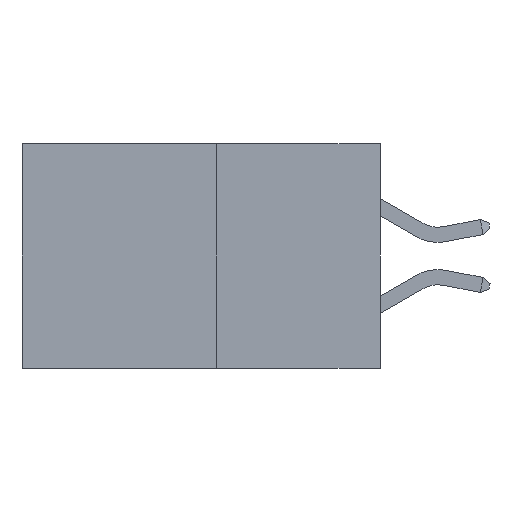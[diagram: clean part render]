
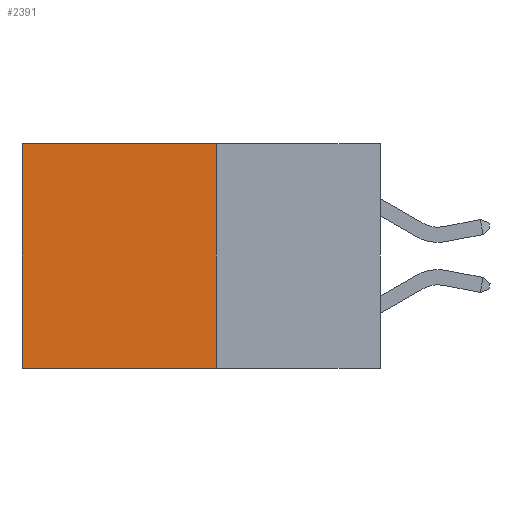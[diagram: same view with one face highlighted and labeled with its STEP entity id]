
A CAD part, left-side view. The second image highlights one B-rep face of the part: STEP entity #2391.
In plain terms, the highlighted planar face has unit normal (-1, 0, 0).
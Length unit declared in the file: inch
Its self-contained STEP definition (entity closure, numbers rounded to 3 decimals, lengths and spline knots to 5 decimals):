
#100 = VERTEX_POINT ( 'NONE', #1561 ) ;
#181 = ORIENTED_EDGE ( 'NONE', *, *, #696, .T. ) ;
#211 = ORIENTED_EDGE ( 'NONE', *, *, #6162, .F. ) ;
#221 = ORIENTED_EDGE ( 'NONE', *, *, #8877, .F. ) ;
#266 = ORIENTED_EDGE ( 'NONE', *, *, #320, .T. ) ;
#320 = EDGE_CURVE ( 'NONE', #9287, #100, #10865, .T. ) ;
#696 = EDGE_CURVE ( 'NONE', #100, #4154, #11442, .T. ) ;
#724 = LINE ( 'NONE', #2511, #7704 ) ;
#786 = VERTEX_POINT ( 'NONE', #1816 ) ;
#1243 = VECTOR ( 'NONE', #10670, 39.37008 ) ;
#1561 = CARTESIAN_POINT ( 'NONE',  ( 0.277, 0.59, 0. ) ) ;
#1816 = CARTESIAN_POINT ( 'NONE',  ( 0.277, 0.27, -0.37 ) ) ;
#2391 = ADVANCED_FACE ( 'NONE', ( #6535 ), #7886, .F. ) ;
#2511 = CARTESIAN_POINT ( 'NONE',  ( 0.277, 0.27, -0.37 ) ) ;
#2722 = DIRECTION ( 'NONE',  ( 1., 0., 0. ) ) ;
#3398 = LINE ( 'NONE', #9887, #5112 ) ;
#3679 = DIRECTION ( 'NONE',  ( 0., 0., -1. ) ) ;
#4154 = VERTEX_POINT ( 'NONE', #10105 ) ;
#5112 = VECTOR ( 'NONE', #10684, 39.37008 ) ;
#5475 = AXIS2_PLACEMENT_3D ( 'NONE', #6475, #2722, #6484 ) ;
#5680 = EDGE_LOOP ( 'NONE', ( #181, #211, #221, #266 ) ) ;
#6162 = EDGE_CURVE ( 'NONE', #786, #4154, #3398, .T. ) ;
#6475 = CARTESIAN_POINT ( 'NONE',  ( 0.277, 0.27, -0.37 ) ) ;
#6484 = DIRECTION ( 'NONE',  ( 0., 0., -1. ) ) ;
#6535 = FACE_OUTER_BOUND ( 'NONE', #5680, .T. ) ;
#7495 = CARTESIAN_POINT ( 'NONE',  ( 0.277, 0.27, 0. ) ) ;
#7704 = VECTOR ( 'NONE', #9703, 39.37008 ) ;
#7886 = PLANE ( 'NONE',  #5475 ) ;
#8877 = EDGE_CURVE ( 'NONE', #9287, #786, #724, .T. ) ;
#9287 = VERTEX_POINT ( 'NONE', #10017 ) ;
#9338 = VECTOR ( 'NONE', #3679, 39.37008 ) ;
#9703 = DIRECTION ( 'NONE',  ( 0., 0., -1. ) ) ;
#9887 = CARTESIAN_POINT ( 'NONE',  ( 0.277, 0.27, -0.37 ) ) ;
#10017 = CARTESIAN_POINT ( 'NONE',  ( 0.277, 0.27, 0. ) ) ;
#10105 = CARTESIAN_POINT ( 'NONE',  ( 0.277, 0.59, -0.37 ) ) ;
#10368 = CARTESIAN_POINT ( 'NONE',  ( 0.277, 0.59, -0.37 ) ) ;
#10670 = DIRECTION ( 'NONE',  ( 0., 1., 0. ) ) ;
#10684 = DIRECTION ( 'NONE',  ( 0., 1., 0. ) ) ;
#10865 = LINE ( 'NONE', #7495, #1243 ) ;
#11442 = LINE ( 'NONE', #10368, #9338 ) ;
